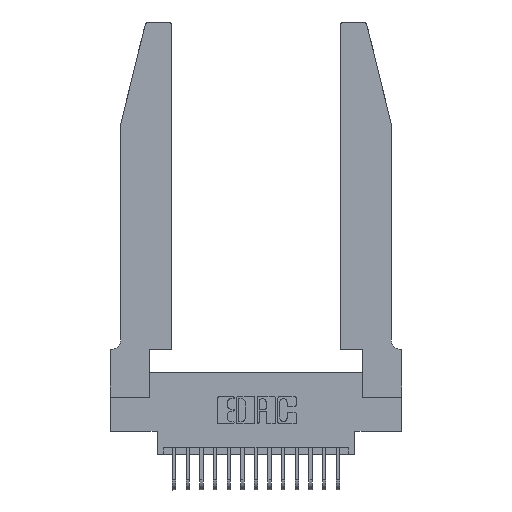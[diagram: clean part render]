
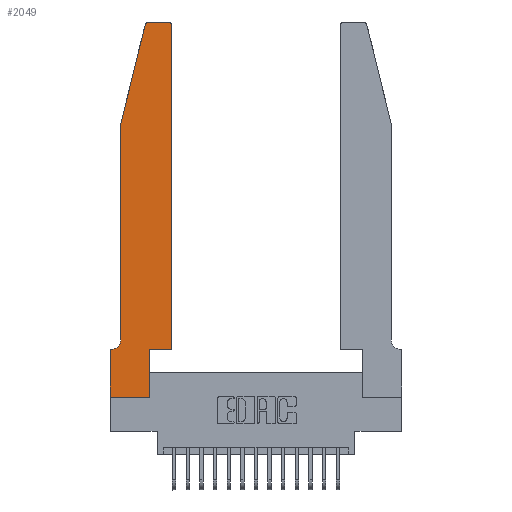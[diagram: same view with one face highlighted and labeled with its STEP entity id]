
A CAD part, top view. The second image highlights one B-rep face of the part: STEP entity #2049.
In plain terms, the highlighted planar face has unit normal (0, 0, 1).
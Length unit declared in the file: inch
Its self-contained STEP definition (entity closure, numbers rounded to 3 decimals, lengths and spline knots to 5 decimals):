
#24 = CARTESIAN_POINT ( 'NONE',  ( 0.2865, 0.35, 0.37 ) ) ;
#82 = LINE ( 'NONE', #8494, #7382 ) ;
#89 = VERTEX_POINT ( 'NONE', #24 ) ;
#325 = LINE ( 'NONE', #6607, #4195 ) ;
#1084 = DIRECTION ( 'NONE',  ( 0., -1., 0. ) ) ;
#1119 = DIRECTION ( 'NONE',  ( 0., 0., 1. ) ) ;
#1125 = VERTEX_POINT ( 'NONE', #5523 ) ;
#1207 = EDGE_CURVE ( 'NONE', #18285, #10030, #325, .T. ) ;
#1214 = LINE ( 'NONE', #9911, #8957 ) ;
#1230 = DIRECTION ( 'NONE',  ( -1., 0., 0. ) ) ;
#1747 = VERTEX_POINT ( 'NONE', #3106 ) ;
#2049 = ADVANCED_FACE ( 'NONE', ( #5101 ), #6104, .T. ) ;
#2114 = CIRCLE ( 'NONE', #3008, 0.03 ) ;
#2531 = EDGE_CURVE ( 'NONE', #10030, #18161, #2114, .T. ) ;
#2654 = VECTOR ( 'NONE', #17196, 39.37008 ) ;
#3008 = AXIS2_PLACEMENT_3D ( 'NONE', #11110, #1119, #10661 ) ;
#3106 = CARTESIAN_POINT ( 'NONE',  ( 0., 0., 0.37 ) ) ;
#3323 = VECTOR ( 'NONE', #8782, 39.37008 ) ;
#4195 = VECTOR ( 'NONE', #6569, 39.37008 ) ;
#4543 = CARTESIAN_POINT ( 'NONE',  ( 0.2865, 0.35, 0.37 ) ) ;
#4898 = VECTOR ( 'NONE', #7478, 39.37008 ) ;
#5101 = FACE_OUTER_BOUND ( 'NONE', #14113, .T. ) ;
#5358 = LINE ( 'NONE', #4543, #4898 ) ;
#5466 = VERTEX_POINT ( 'NONE', #14050 ) ;
#5493 = ORIENTED_EDGE ( 'NONE', *, *, #18338, .T. ) ;
#5523 = CARTESIAN_POINT ( 'NONE',  ( 0.25487, 2.72718, 0.37 ) ) ;
#5652 = EDGE_CURVE ( 'NONE', #89, #18285, #13832, .T. ) ;
#5737 = ORIENTED_EDGE ( 'NONE', *, *, #5652, .T. ) ;
#5873 = DIRECTION ( 'NONE',  ( 1., 0., 0. ) ) ;
#5943 = DIRECTION ( 'NONE',  ( 0., 0., 1. ) ) ;
#5969 = DIRECTION ( 'NONE',  ( 1., 0., 0. ) ) ;
#6030 = VERTEX_POINT ( 'NONE', #12813 ) ;
#6104 = PLANE ( 'NONE',  #17274 ) ;
#6132 = VECTOR ( 'NONE', #5873, 39.37008 ) ;
#6241 = CARTESIAN_POINT ( 'NONE',  ( 0.284, 2.72, 0.37 ) ) ;
#6316 = CARTESIAN_POINT ( 'NONE',  ( 0.0055, 0.35, 0.37 ) ) ;
#6386 = DIRECTION ( 'NONE',  ( 0., 0., -1. ) ) ;
#6569 = DIRECTION ( 'NONE',  ( 0., 1., 0. ) ) ;
#6607 = CARTESIAN_POINT ( 'NONE',  ( 0.4505, 0.35, 0.37 ) ) ;
#6942 = EDGE_CURVE ( 'NONE', #6030, #18639, #9694, .T. ) ;
#7120 = EDGE_CURVE ( 'NONE', #16740, #1747, #9906, .T. ) ;
#7292 = EDGE_CURVE ( 'NONE', #1125, #11275, #14887, .T. ) ;
#7320 = CARTESIAN_POINT ( 'NONE',  ( 0.0755, 2., 0.37 ) ) ;
#7382 = VECTOR ( 'NONE', #1230, 39.37008 ) ;
#7478 = DIRECTION ( 'NONE',  ( 0., 1., 0. ) ) ;
#7511 = ORIENTED_EDGE ( 'NONE', *, *, #10304, .T. ) ;
#7630 = CARTESIAN_POINT ( 'NONE',  ( 0.4205, 2.75, 0.37 ) ) ;
#7694 = DIRECTION ( 'NONE',  ( 1., 0., 0. ) ) ;
#8155 = ORIENTED_EDGE ( 'NONE', *, *, #6942, .T. ) ;
#8430 = EDGE_CURVE ( 'NONE', #18639, #16740, #82, .T. ) ;
#8494 = CARTESIAN_POINT ( 'NONE',  ( 0.0755, 0.35, 0.37 ) ) ;
#8782 = DIRECTION ( 'NONE',  ( -0.239, -0.971, 0. ) ) ;
#8957 = VECTOR ( 'NONE', #12844, 39.37008 ) ;
#9451 = ORIENTED_EDGE ( 'NONE', *, *, #17630, .T. ) ;
#9629 = AXIS2_PLACEMENT_3D ( 'NONE', #15029, #6386, #16461 ) ;
#9694 = CIRCLE ( 'NONE', #9629, 0.07 ) ;
#9906 = LINE ( 'NONE', #18337, #17102 ) ;
#9911 = CARTESIAN_POINT ( 'NONE',  ( 0.0755, 2., 0.37 ) ) ;
#10030 = VERTEX_POINT ( 'NONE', #17130 ) ;
#10304 = EDGE_CURVE ( 'NONE', #13873, #1125, #13047, .T. ) ;
#10407 = VECTOR ( 'NONE', #12887, 39.37008 ) ;
#10417 = ORIENTED_EDGE ( 'NONE', *, *, #7292, .T. ) ;
#10661 = DIRECTION ( 'NONE',  ( 1., 0., 0. ) ) ;
#10883 = LINE ( 'NONE', #11446, #10407 ) ;
#11110 = CARTESIAN_POINT ( 'NONE',  ( 0.4205, 2.72, 0.37 ) ) ;
#11275 = VERTEX_POINT ( 'NONE', #15350 ) ;
#11446 = CARTESIAN_POINT ( 'NONE',  ( 0., 0., 0.37 ) ) ;
#11536 = CARTESIAN_POINT ( 'NONE',  ( 0.2605, 2.75, 0.37 ) ) ;
#12522 = CARTESIAN_POINT ( 'NONE',  ( 0.284, 2.75, 0.37 ) ) ;
#12813 = CARTESIAN_POINT ( 'NONE',  ( 0.0755, 0.42, 0.37 ) ) ;
#12844 = DIRECTION ( 'NONE',  ( 0., -1., 0. ) ) ;
#12887 = DIRECTION ( 'NONE',  ( 1., 0., 0. ) ) ;
#13047 = CIRCLE ( 'NONE', #13813, 0.03 ) ;
#13798 = ORIENTED_EDGE ( 'NONE', *, *, #15905, .T. ) ;
#13813 = AXIS2_PLACEMENT_3D ( 'NONE', #6241, #16320, #7694 ) ;
#13832 = LINE ( 'NONE', #17388, #6132 ) ;
#13871 = ORIENTED_EDGE ( 'NONE', *, *, #14684, .T. ) ;
#13873 = VERTEX_POINT ( 'NONE', #12522 ) ;
#14050 = CARTESIAN_POINT ( 'NONE',  ( 0.2865, 0., 0.37 ) ) ;
#14113 = EDGE_LOOP ( 'NONE', ( #13798, #7511, #10417, #5493, #8155, #14616, #15671, #13871, #9451, #5737, #15670, #17313 ) ) ;
#14250 = LINE ( 'NONE', #11536, #2654 ) ;
#14616 = ORIENTED_EDGE ( 'NONE', *, *, #8430, .T. ) ;
#14684 = EDGE_CURVE ( 'NONE', #1747, #5466, #10883, .T. ) ;
#14887 = LINE ( 'NONE', #7320, #3323 ) ;
#15029 = CARTESIAN_POINT ( 'NONE',  ( 0.0055, 0.42, 0.37 ) ) ;
#15350 = CARTESIAN_POINT ( 'NONE',  ( 0.0755, 2., 0.37 ) ) ;
#15670 = ORIENTED_EDGE ( 'NONE', *, *, #1207, .T. ) ;
#15671 = ORIENTED_EDGE ( 'NONE', *, *, #7120, .T. ) ;
#15905 = EDGE_CURVE ( 'NONE', #18161, #13873, #14250, .T. ) ;
#16320 = DIRECTION ( 'NONE',  ( 0., 0., 1. ) ) ;
#16461 = DIRECTION ( 'NONE',  ( -1., 0., 0. ) ) ;
#16510 = CARTESIAN_POINT ( 'NONE',  ( 0.4505, 0.35, 0.37 ) ) ;
#16740 = VERTEX_POINT ( 'NONE', #17665 ) ;
#17102 = VECTOR ( 'NONE', #1084, 39.37008 ) ;
#17130 = CARTESIAN_POINT ( 'NONE',  ( 0.4505, 2.72, 0.37 ) ) ;
#17196 = DIRECTION ( 'NONE',  ( -1., 0., 0. ) ) ;
#17274 = AXIS2_PLACEMENT_3D ( 'NONE', #18127, #5943, #5969 ) ;
#17313 = ORIENTED_EDGE ( 'NONE', *, *, #2531, .T. ) ;
#17388 = CARTESIAN_POINT ( 'NONE',  ( 0.4505, 0.35, 0.37 ) ) ;
#17630 = EDGE_CURVE ( 'NONE', #5466, #89, #5358, .T. ) ;
#17665 = CARTESIAN_POINT ( 'NONE',  ( 0., 0.35, 0.37 ) ) ;
#18127 = CARTESIAN_POINT ( 'NONE',  ( 0., 0.35, 0.37 ) ) ;
#18161 = VERTEX_POINT ( 'NONE', #7630 ) ;
#18285 = VERTEX_POINT ( 'NONE', #16510 ) ;
#18337 = CARTESIAN_POINT ( 'NONE',  ( 0., 0., 0.37 ) ) ;
#18338 = EDGE_CURVE ( 'NONE', #11275, #6030, #1214, .T. ) ;
#18639 = VERTEX_POINT ( 'NONE', #6316 ) ;
